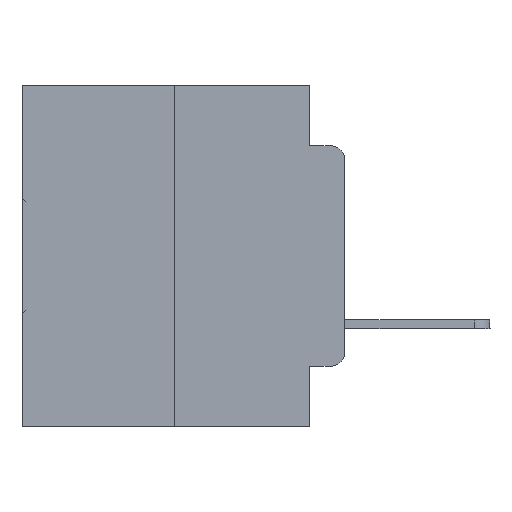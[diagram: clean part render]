
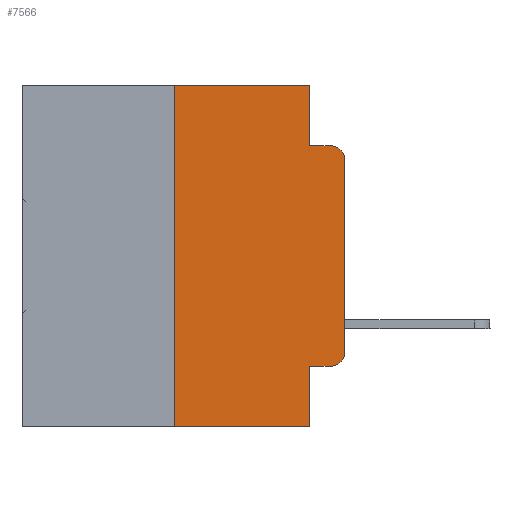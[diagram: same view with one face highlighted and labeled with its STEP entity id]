
A CAD part, left-side view. The second image highlights one B-rep face of the part: STEP entity #7566.
In plain terms, the highlighted planar face has unit normal (-1, 0, 0).
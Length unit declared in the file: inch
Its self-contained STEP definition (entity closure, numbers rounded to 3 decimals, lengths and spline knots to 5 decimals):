
#141 = ORIENTED_EDGE ( 'NONE', *, *, #18099, .F. ) ;
#1169 = FACE_OUTER_BOUND ( 'NONE', #26135, .T. ) ;
#1555 = CIRCLE ( 'NONE', #8264, 0.02 ) ;
#1795 = ORIENTED_EDGE ( 'NONE', *, *, #22854, .T. ) ;
#1950 = ORIENTED_EDGE ( 'NONE', *, *, #14653, .T. ) ;
#2179 = ORIENTED_EDGE ( 'NONE', *, *, #12260, .T. ) ;
#2569 = VECTOR ( 'NONE', #13344, 39.37008 ) ;
#2739 = LINE ( 'NONE', #21107, #16793 ) ;
#4077 = ORIENTED_EDGE ( 'NONE', *, *, #13655, .F. ) ;
#4928 = CARTESIAN_POINT ( 'NONE',  ( 0., 0.051, -0.4115 ) ) ;
#5131 = CARTESIAN_POINT ( 'NONE',  ( 0., 0.051, -0.5 ) ) ;
#5194 = LINE ( 'NONE', #30937, #29410 ) ;
#5650 = CARTESIAN_POINT ( 'NONE',  ( 0., 0.051, 0. ) ) ;
#6858 = ORIENTED_EDGE ( 'NONE', *, *, #29916, .F. ) ;
#7374 = LINE ( 'NONE', #4928, #25976 ) ;
#7566 = ADVANCED_FACE ( 'NONE', ( #1169 ), #14328, .F. ) ;
#7788 = CARTESIAN_POINT ( 'NONE',  ( 0., 0.051, -0.4115 ) ) ;
#8264 = AXIS2_PLACEMENT_3D ( 'NONE', #19027, #26118, #16620 ) ;
#8514 = CARTESIAN_POINT ( 'NONE',  ( 0., 0.02, -0.3915 ) ) ;
#8621 = EDGE_CURVE ( 'NONE', #24695, #31160, #5194, .T. ) ;
#8848 = CARTESIAN_POINT ( 'NONE',  ( 0., 0.051, -0.0885 ) ) ;
#8883 = CARTESIAN_POINT ( 'NONE',  ( 0., 0.25, 0. ) ) ;
#9004 = LINE ( 'NONE', #15238, #2569 ) ;
#9093 = DIRECTION ( 'NONE',  ( 0., 0., 1. ) ) ;
#9263 = DIRECTION ( 'NONE',  ( 0., -1., 0. ) ) ;
#9960 = AXIS2_PLACEMENT_3D ( 'NONE', #8514, #16089, #30207 ) ;
#10194 = VERTEX_POINT ( 'NONE', #8848 ) ;
#10363 = DIRECTION ( 'NONE',  ( 0., 0., -1. ) ) ;
#10494 = VECTOR ( 'NONE', #29117, 39.37008 ) ;
#10638 = CARTESIAN_POINT ( 'NONE',  ( 0., 0.473, 0. ) ) ;
#11059 = ORIENTED_EDGE ( 'NONE', *, *, #16822, .T. ) ;
#11549 = DIRECTION ( 'NONE',  ( 0., -1., 0. ) ) ;
#12260 = EDGE_CURVE ( 'NONE', #31160, #19997, #1555, .T. ) ;
#13334 = DIRECTION ( 'NONE',  ( 0., 0., -1. ) ) ;
#13344 = DIRECTION ( 'NONE',  ( 0., -1., 0. ) ) ;
#13580 = VERTEX_POINT ( 'NONE', #5131 ) ;
#13590 = LINE ( 'NONE', #14758, #10494 ) ;
#13655 = EDGE_CURVE ( 'NONE', #20935, #13580, #13590, .T. ) ;
#14178 = CARTESIAN_POINT ( 'NONE',  ( 0., 0.051, -0.0885 ) ) ;
#14328 = PLANE ( 'NONE',  #27291 ) ;
#14494 = LINE ( 'NONE', #8883, #29580 ) ;
#14653 = EDGE_CURVE ( 'NONE', #20935, #25810, #7374, .T. ) ;
#14758 = CARTESIAN_POINT ( 'NONE',  ( 0., 0.051, 0. ) ) ;
#15238 = CARTESIAN_POINT ( 'NONE',  ( 0., 0.473, -0.5 ) ) ;
#15378 = CARTESIAN_POINT ( 'NONE',  ( 0., 0.051, 0. ) ) ;
#15688 = CARTESIAN_POINT ( 'NONE',  ( 0., 0.25, 0. ) ) ;
#16089 = DIRECTION ( 'NONE',  ( -1., 0., 0. ) ) ;
#16317 = LINE ( 'NONE', #14178, #21201 ) ;
#16620 = DIRECTION ( 'NONE',  ( 0., 0., -1. ) ) ;
#16793 = VECTOR ( 'NONE', #11549, 39.37008 ) ;
#16822 = EDGE_CURVE ( 'NONE', #25810, #24695, #21310, .T. ) ;
#18099 = EDGE_CURVE ( 'NONE', #19235, #10194, #30463, .T. ) ;
#18105 = DIRECTION ( 'NONE',  ( 1., 0., 0. ) ) ;
#18802 = DIRECTION ( 'NONE',  ( 0., 0., 1. ) ) ;
#18830 = VERTEX_POINT ( 'NONE', #15688 ) ;
#19027 = CARTESIAN_POINT ( 'NONE',  ( 0., 0.02, -0.1085 ) ) ;
#19235 = VERTEX_POINT ( 'NONE', #5650 ) ;
#19249 = ORIENTED_EDGE ( 'NONE', *, *, #25876, .F. ) ;
#19649 = VERTEX_POINT ( 'NONE', #24060 ) ;
#19997 = VERTEX_POINT ( 'NONE', #27723 ) ;
#20047 = EDGE_CURVE ( 'NONE', #18830, #19235, #2739, .T. ) ;
#20629 = VECTOR ( 'NONE', #10363, 39.37008 ) ;
#20935 = VERTEX_POINT ( 'NONE', #7788 ) ;
#21107 = CARTESIAN_POINT ( 'NONE',  ( 0., 0.473, 0. ) ) ;
#21201 = VECTOR ( 'NONE', #9263, 39.37008 ) ;
#21310 = CIRCLE ( 'NONE', #9960, 0.02 ) ;
#21845 = DIRECTION ( 'NONE',  ( 0., -1., 0. ) ) ;
#22854 = EDGE_CURVE ( 'NONE', #19649, #13580, #9004, .T. ) ;
#24060 = CARTESIAN_POINT ( 'NONE',  ( 0., 0.25, -0.5 ) ) ;
#24695 = VERTEX_POINT ( 'NONE', #26182 ) ;
#25810 = VERTEX_POINT ( 'NONE', #28332 ) ;
#25876 = EDGE_CURVE ( 'NONE', #10194, #19997, #16317, .T. ) ;
#25976 = VECTOR ( 'NONE', #21845, 39.37008 ) ;
#26018 = ORIENTED_EDGE ( 'NONE', *, *, #8621, .T. ) ;
#26118 = DIRECTION ( 'NONE',  ( -1., 0., 0. ) ) ;
#26135 = EDGE_LOOP ( 'NONE', ( #26018, #2179, #19249, #141, #31154, #6858, #1795, #4077, #1950, #11059 ) ) ;
#26182 = CARTESIAN_POINT ( 'NONE',  ( 0., 0., -0.3915 ) ) ;
#27291 = AXIS2_PLACEMENT_3D ( 'NONE', #10638, #18105, #13334 ) ;
#27723 = CARTESIAN_POINT ( 'NONE',  ( 0., 0.02, -0.0885 ) ) ;
#28332 = CARTESIAN_POINT ( 'NONE',  ( 0., 0.02, -0.4115 ) ) ;
#28492 = CARTESIAN_POINT ( 'NONE',  ( 0., 0., -0.1085 ) ) ;
#29117 = DIRECTION ( 'NONE',  ( 0., 0., -1. ) ) ;
#29410 = VECTOR ( 'NONE', #18802, 39.37008 ) ;
#29580 = VECTOR ( 'NONE', #9093, 39.37008 ) ;
#29916 = EDGE_CURVE ( 'NONE', #19649, #18830, #14494, .T. ) ;
#30207 = DIRECTION ( 'NONE',  ( 0., 0., -1. ) ) ;
#30463 = LINE ( 'NONE', #15378, #20629 ) ;
#30937 = CARTESIAN_POINT ( 'NONE',  ( 0., 0., 0. ) ) ;
#31154 = ORIENTED_EDGE ( 'NONE', *, *, #20047, .F. ) ;
#31160 = VERTEX_POINT ( 'NONE', #28492 ) ;
